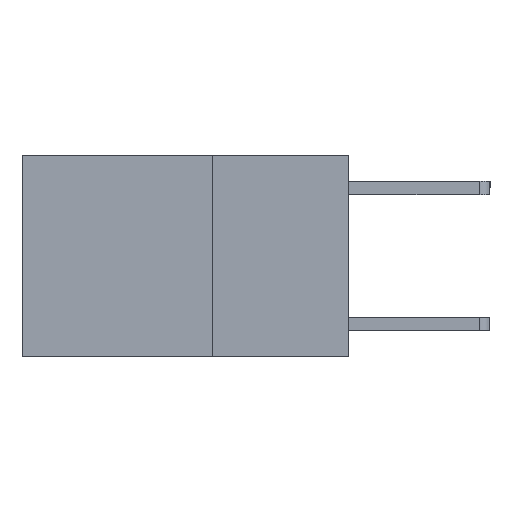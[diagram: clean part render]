
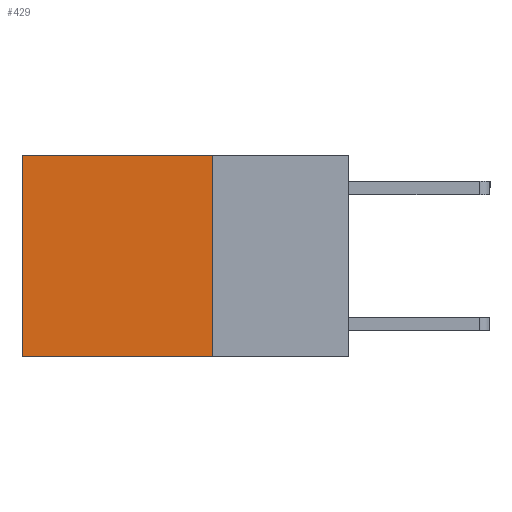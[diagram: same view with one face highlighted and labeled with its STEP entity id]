
A CAD part, left-side view. The second image highlights one B-rep face of the part: STEP entity #429.
In plain terms, the highlighted planar face has unit normal (-1, 0, 0).
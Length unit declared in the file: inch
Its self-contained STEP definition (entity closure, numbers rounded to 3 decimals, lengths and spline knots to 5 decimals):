
#360 = DIRECTION ( 'NONE',  ( 0., 0., -1. ) ) ;
#429 = ADVANCED_FACE ( 'NONE', ( #4083 ), #11015, .F. ) ;
#893 = EDGE_CURVE ( 'NONE', #10699, #10740, #7345, .T. ) ;
#1330 = ORIENTED_EDGE ( 'NONE', *, *, #7667, .T. ) ;
#1429 = EDGE_CURVE ( 'NONE', #10699, #9167, #10279, .T. ) ;
#1781 = DIRECTION ( 'NONE',  ( 0., 0., -1. ) ) ;
#1884 = VERTEX_POINT ( 'NONE', #9042 ) ;
#2121 = DIRECTION ( 'NONE',  ( 1., 0., 0. ) ) ;
#2305 = DIRECTION ( 'NONE',  ( 0., 1., 0. ) ) ;
#2727 = CARTESIAN_POINT ( 'NONE',  ( 0.2625, 0.6, 0. ) ) ;
#2919 = VECTOR ( 'NONE', #1781, 39.37008 ) ;
#3040 = ORIENTED_EDGE ( 'NONE', *, *, #893, .F. ) ;
#3180 = CARTESIAN_POINT ( 'NONE',  ( 0.2625, 0.25, 0. ) ) ;
#4083 = FACE_OUTER_BOUND ( 'NONE', #7342, .T. ) ;
#4431 = CARTESIAN_POINT ( 'NONE',  ( 0.2625, 0.25, -0.37 ) ) ;
#5460 = DIRECTION ( 'NONE',  ( 0., 0., -1. ) ) ;
#5505 = VECTOR ( 'NONE', #7413, 39.37008 ) ;
#6002 = EDGE_CURVE ( 'NONE', #10740, #1884, #11059, .T. ) ;
#7211 = CARTESIAN_POINT ( 'NONE',  ( 0.2625, 0.25, 0. ) ) ;
#7342 = EDGE_LOOP ( 'NONE', ( #1330, #11919, #3040, #11154 ) ) ;
#7345 = LINE ( 'NONE', #7211, #9498 ) ;
#7413 = DIRECTION ( 'NONE',  ( 0., 1., 0. ) ) ;
#7661 = AXIS2_PLACEMENT_3D ( 'NONE', #3180, #2121, #360 ) ;
#7667 = EDGE_CURVE ( 'NONE', #9167, #1884, #8539, .T. ) ;
#8288 = CARTESIAN_POINT ( 'NONE',  ( 0.2625, 0.25, -0.37 ) ) ;
#8539 = LINE ( 'NONE', #2727, #2919 ) ;
#9042 = CARTESIAN_POINT ( 'NONE',  ( 0.2625, 0.6, -0.37 ) ) ;
#9167 = VERTEX_POINT ( 'NONE', #11869 ) ;
#9498 = VECTOR ( 'NONE', #5460, 39.37008 ) ;
#10279 = LINE ( 'NONE', #11084, #11171 ) ;
#10524 = CARTESIAN_POINT ( 'NONE',  ( 0.2625, 0.25, 0. ) ) ;
#10699 = VERTEX_POINT ( 'NONE', #10524 ) ;
#10740 = VERTEX_POINT ( 'NONE', #4431 ) ;
#11015 = PLANE ( 'NONE',  #7661 ) ;
#11059 = LINE ( 'NONE', #8288, #5505 ) ;
#11084 = CARTESIAN_POINT ( 'NONE',  ( 0.2625, 0.25, 0. ) ) ;
#11154 = ORIENTED_EDGE ( 'NONE', *, *, #1429, .T. ) ;
#11171 = VECTOR ( 'NONE', #2305, 39.37008 ) ;
#11869 = CARTESIAN_POINT ( 'NONE',  ( 0.2625, 0.6, 0. ) ) ;
#11919 = ORIENTED_EDGE ( 'NONE', *, *, #6002, .F. ) ;
